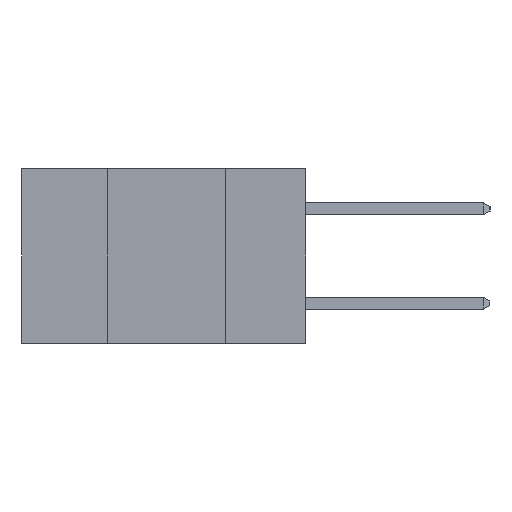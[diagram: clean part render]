
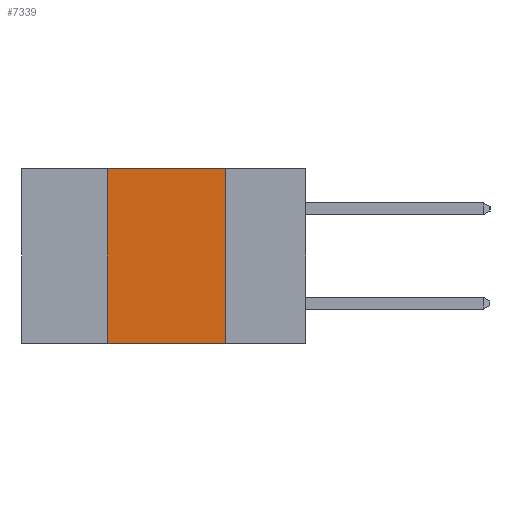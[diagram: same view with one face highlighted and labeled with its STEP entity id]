
A CAD part, left-side view. The second image highlights one B-rep face of the part: STEP entity #7339.
In plain terms, the highlighted planar face has unit normal (-1, 0, 0).
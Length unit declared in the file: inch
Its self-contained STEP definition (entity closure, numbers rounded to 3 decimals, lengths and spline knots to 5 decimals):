
#83 = VERTEX_POINT ( 'NONE', #15049 ) ;
#267 = LINE ( 'NONE', #8240, #1148 ) ;
#401 = AXIS2_PLACEMENT_3D ( 'NONE', #8263, #2491, #15638 ) ;
#528 = FACE_OUTER_BOUND ( 'NONE', #11228, .T. ) ;
#851 = DIRECTION ( 'NONE',  ( 0., -1., 0. ) ) ;
#1115 = CARTESIAN_POINT ( 'NONE',  ( 0., 0.17, 0. ) ) ;
#1148 = VECTOR ( 'NONE', #10581, 39.37008 ) ;
#1208 = VECTOR ( 'NONE', #15878, 39.37008 ) ;
#2491 = DIRECTION ( 'NONE',  ( 1., 0., 0. ) ) ;
#3516 = LINE ( 'NONE', #3644, #15622 ) ;
#3644 = CARTESIAN_POINT ( 'NONE',  ( 0., 0.6, -0.37 ) ) ;
#4445 = PLANE ( 'NONE',  #401 ) ;
#7007 = ORIENTED_EDGE ( 'NONE', *, *, #14631, .F. ) ;
#7215 = DIRECTION ( 'NONE',  ( 0., -1., 0. ) ) ;
#7339 = ADVANCED_FACE ( 'NONE', ( #528 ), #4445, .F. ) ;
#8240 = CARTESIAN_POINT ( 'NONE',  ( 0., 0.42, -0.37 ) ) ;
#8263 = CARTESIAN_POINT ( 'NONE',  ( 0., 0.6, 0. ) ) ;
#8375 = LINE ( 'NONE', #16245, #1208 ) ;
#8511 = EDGE_CURVE ( 'NONE', #23577, #83, #3516, .T. ) ;
#10123 = CARTESIAN_POINT ( 'NONE',  ( 0., 0.42, -0.37 ) ) ;
#10495 = CARTESIAN_POINT ( 'NONE',  ( 0., 0.42, 0. ) ) ;
#10581 = DIRECTION ( 'NONE',  ( 0., 0., 1. ) ) ;
#11228 = EDGE_LOOP ( 'NONE', ( #7007, #20727, #17470, #15796 ) ) ;
#12633 = VERTEX_POINT ( 'NONE', #1115 ) ;
#14118 = LINE ( 'NONE', #17680, #16149 ) ;
#14631 = EDGE_CURVE ( 'NONE', #12633, #83, #8375, .T. ) ;
#14642 = EDGE_CURVE ( 'NONE', #23721, #12633, #14118, .T. ) ;
#15049 = CARTESIAN_POINT ( 'NONE',  ( 0., 0.17, -0.37 ) ) ;
#15622 = VECTOR ( 'NONE', #7215, 39.37008 ) ;
#15638 = DIRECTION ( 'NONE',  ( 0., 0., -1. ) ) ;
#15796 = ORIENTED_EDGE ( 'NONE', *, *, #8511, .T. ) ;
#15878 = DIRECTION ( 'NONE',  ( 0., 0., -1. ) ) ;
#16149 = VECTOR ( 'NONE', #851, 39.37008 ) ;
#16245 = CARTESIAN_POINT ( 'NONE',  ( 0., 0.17, -0.37 ) ) ;
#17470 = ORIENTED_EDGE ( 'NONE', *, *, #22799, .F. ) ;
#17680 = CARTESIAN_POINT ( 'NONE',  ( 0., 0.6, 0. ) ) ;
#20727 = ORIENTED_EDGE ( 'NONE', *, *, #14642, .F. ) ;
#22799 = EDGE_CURVE ( 'NONE', #23577, #23721, #267, .T. ) ;
#23577 = VERTEX_POINT ( 'NONE', #10123 ) ;
#23721 = VERTEX_POINT ( 'NONE', #10495 ) ;
